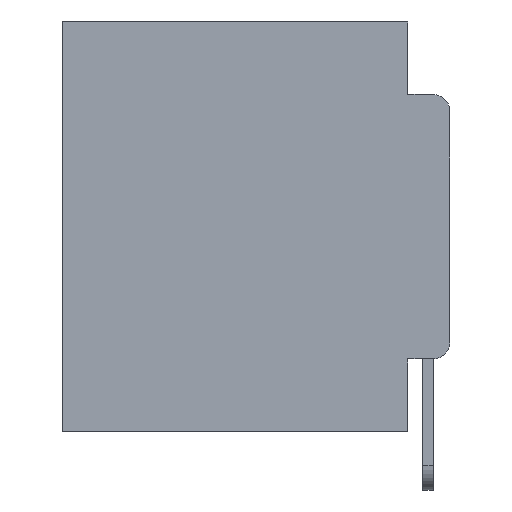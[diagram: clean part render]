
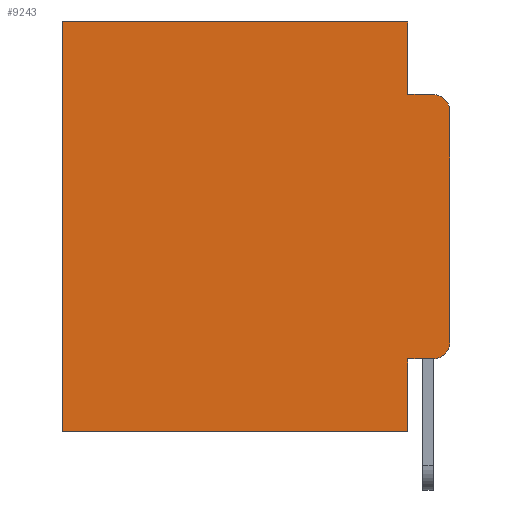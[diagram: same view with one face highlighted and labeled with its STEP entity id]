
A CAD part, left-side view. The second image highlights one B-rep face of the part: STEP entity #9243.
In plain terms, the highlighted planar face has unit normal (-1, 0, 0).
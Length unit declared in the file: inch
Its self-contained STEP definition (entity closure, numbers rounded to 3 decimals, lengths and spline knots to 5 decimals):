
#217 = LINE ( 'NONE', #2823, #7219 ) ;
#425 = DIRECTION ( 'NONE',  ( 0., -1., 0. ) ) ;
#2062 = ORIENTED_EDGE ( 'NONE', *, *, #9405, .F. ) ;
#2558 = LINE ( 'NONE', #27913, #19277 ) ;
#2658 = CARTESIAN_POINT ( 'NONE',  ( 0.298, 0., -0.3915 ) ) ;
#2823 = CARTESIAN_POINT ( 'NONE',  ( 0.298, 0., 0. ) ) ;
#3448 = VECTOR ( 'NONE', #6583, 39.37008 ) ;
#5059 = ORIENTED_EDGE ( 'NONE', *, *, #14928, .T. ) ;
#5537 = VECTOR ( 'NONE', #18974, 39.37008 ) ;
#5539 = VECTOR ( 'NONE', #18236, 39.37008 ) ;
#6249 = LINE ( 'NONE', #11611, #5539 ) ;
#6515 = ORIENTED_EDGE ( 'NONE', *, *, #20823, .T. ) ;
#6524 = EDGE_LOOP ( 'NONE', ( #2062, #5059, #7602, #27062, #26721, #10505, #24702, #6545, #19248, #6515 ) ) ;
#6545 = ORIENTED_EDGE ( 'NONE', *, *, #9075, .F. ) ;
#6583 = DIRECTION ( 'NONE',  ( 0., 0., -1. ) ) ;
#6865 = FACE_OUTER_BOUND ( 'NONE', #6524, .T. ) ;
#7219 = VECTOR ( 'NONE', #16546, 39.37008 ) ;
#7462 = EDGE_CURVE ( 'NONE', #14228, #22228, #6249, .T. ) ;
#7544 = CARTESIAN_POINT ( 'NONE',  ( 0.298, 0.051, -0.4115 ) ) ;
#7602 = ORIENTED_EDGE ( 'NONE', *, *, #7462, .F. ) ;
#7963 = LINE ( 'NONE', #16445, #24317 ) ;
#8500 = CIRCLE ( 'NONE', #9896, 0.02 ) ;
#8556 = VERTEX_POINT ( 'NONE', #11478 ) ;
#9075 = EDGE_CURVE ( 'NONE', #16128, #26527, #22981, .T. ) ;
#9243 = ADVANCED_FACE ( 'NONE', ( #6865 ), #11435, .F. ) ;
#9275 = CARTESIAN_POINT ( 'NONE',  ( 0.298, 0.051, 0. ) ) ;
#9405 = EDGE_CURVE ( 'NONE', #8556, #16049, #217, .T. ) ;
#9546 = CARTESIAN_POINT ( 'NONE',  ( 0.298, 0.051, -0.0885 ) ) ;
#9826 = CARTESIAN_POINT ( 'NONE',  ( 0.298, 0.02, -0.0885 ) ) ;
#9896 = AXIS2_PLACEMENT_3D ( 'NONE', #12552, #27889, #14794 ) ;
#10349 = LINE ( 'NONE', #17882, #3448 ) ;
#10505 = ORIENTED_EDGE ( 'NONE', *, *, #25904, .T. ) ;
#11215 = VECTOR ( 'NONE', #17595, 39.37008 ) ;
#11435 = PLANE ( 'NONE',  #27758 ) ;
#11478 = CARTESIAN_POINT ( 'NONE',  ( 0.298, 0., -0.1085 ) ) ;
#11611 = CARTESIAN_POINT ( 'NONE',  ( 0.298, 0.051, -0.0885 ) ) ;
#12552 = CARTESIAN_POINT ( 'NONE',  ( 0.298, 0.02, -0.1085 ) ) ;
#13310 = VERTEX_POINT ( 'NONE', #9275 ) ;
#13477 = CARTESIAN_POINT ( 'NONE',  ( 0.298, 0.02, -0.3915 ) ) ;
#14228 = VERTEX_POINT ( 'NONE', #9546 ) ;
#14649 = VERTEX_POINT ( 'NONE', #29151 ) ;
#14760 = AXIS2_PLACEMENT_3D ( 'NONE', #13477, #28809, #15742 ) ;
#14794 = DIRECTION ( 'NONE',  ( 0., 0., -1. ) ) ;
#14928 = EDGE_CURVE ( 'NONE', #8556, #22228, #8500, .T. ) ;
#15379 = CARTESIAN_POINT ( 'NONE',  ( 0.298, 0.051, 0. ) ) ;
#15742 = DIRECTION ( 'NONE',  ( 0., 0., -1. ) ) ;
#15932 = CARTESIAN_POINT ( 'NONE',  ( 0.298, 0.02, -0.4115 ) ) ;
#15956 = DIRECTION ( 'NONE',  ( 0., 0., -1. ) ) ;
#16049 = VERTEX_POINT ( 'NONE', #2658 ) ;
#16128 = VERTEX_POINT ( 'NONE', #7544 ) ;
#16445 = CARTESIAN_POINT ( 'NONE',  ( 0.298, 0., -0.5 ) ) ;
#16546 = DIRECTION ( 'NONE',  ( 0., 0., -1. ) ) ;
#16587 = CIRCLE ( 'NONE', #14760, 0.02 ) ;
#17593 = CARTESIAN_POINT ( 'NONE',  ( 0.298, 0.473, -0.5 ) ) ;
#17595 = DIRECTION ( 'NONE',  ( 0., 0., -1. ) ) ;
#17882 = CARTESIAN_POINT ( 'NONE',  ( 0.298, 0.051, 0. ) ) ;
#18068 = CARTESIAN_POINT ( 'NONE',  ( 0.298, 0., 0. ) ) ;
#18236 = DIRECTION ( 'NONE',  ( 0., -1., 0. ) ) ;
#18275 = EDGE_CURVE ( 'NONE', #13310, #14228, #10349, .T. ) ;
#18770 = CARTESIAN_POINT ( 'NONE',  ( 0.298, 0.051, -0.4115 ) ) ;
#18864 = VERTEX_POINT ( 'NONE', #15932 ) ;
#18974 = DIRECTION ( 'NONE',  ( 0., 1., 0. ) ) ;
#18995 = LINE ( 'NONE', #21056, #5537 ) ;
#19248 = ORIENTED_EDGE ( 'NONE', *, *, #21661, .T. ) ;
#19277 = VECTOR ( 'NONE', #28012, 39.37008 ) ;
#19689 = CARTESIAN_POINT ( 'NONE',  ( 0.298, 0.051, -0.5 ) ) ;
#19899 = EDGE_CURVE ( 'NONE', #13310, #14649, #18995, .T. ) ;
#20823 = EDGE_CURVE ( 'NONE', #18864, #16049, #16587, .T. ) ;
#21056 = CARTESIAN_POINT ( 'NONE',  ( 0.298, 0., 0. ) ) ;
#21661 = EDGE_CURVE ( 'NONE', #16128, #18864, #26747, .T. ) ;
#22228 = VERTEX_POINT ( 'NONE', #9826 ) ;
#22981 = LINE ( 'NONE', #15379, #11215 ) ;
#24317 = VECTOR ( 'NONE', #27302, 39.37008 ) ;
#24702 = ORIENTED_EDGE ( 'NONE', *, *, #26820, .F. ) ;
#25904 = EDGE_CURVE ( 'NONE', #14649, #26553, #2558, .T. ) ;
#26073 = VECTOR ( 'NONE', #425, 39.37008 ) ;
#26527 = VERTEX_POINT ( 'NONE', #19689 ) ;
#26553 = VERTEX_POINT ( 'NONE', #17593 ) ;
#26721 = ORIENTED_EDGE ( 'NONE', *, *, #19899, .T. ) ;
#26747 = LINE ( 'NONE', #18770, #26073 ) ;
#26820 = EDGE_CURVE ( 'NONE', #26527, #26553, #7963, .T. ) ;
#27062 = ORIENTED_EDGE ( 'NONE', *, *, #18275, .F. ) ;
#27302 = DIRECTION ( 'NONE',  ( 0., 1., 0. ) ) ;
#27758 = AXIS2_PLACEMENT_3D ( 'NONE', #18068, #29024, #15956 ) ;
#27889 = DIRECTION ( 'NONE',  ( -1., 0., 0. ) ) ;
#27913 = CARTESIAN_POINT ( 'NONE',  ( 0.298, 0.473, 0. ) ) ;
#28012 = DIRECTION ( 'NONE',  ( 0., 0., -1. ) ) ;
#28809 = DIRECTION ( 'NONE',  ( -1., 0., 0. ) ) ;
#29024 = DIRECTION ( 'NONE',  ( 1., 0., 0. ) ) ;
#29151 = CARTESIAN_POINT ( 'NONE',  ( 0.298, 0.473, 0. ) ) ;
